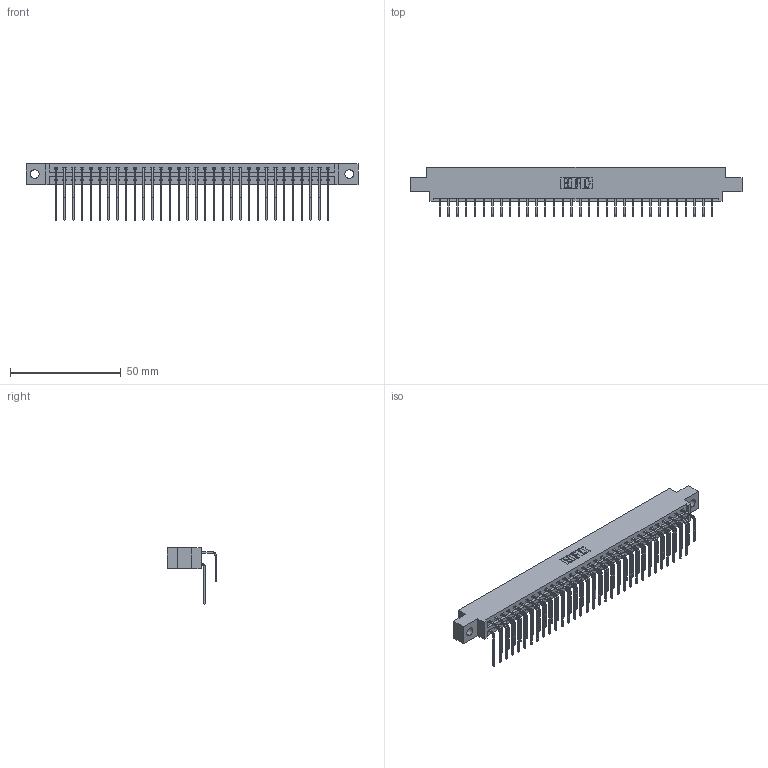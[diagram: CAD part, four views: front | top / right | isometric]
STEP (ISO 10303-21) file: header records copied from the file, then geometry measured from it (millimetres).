
FILE_DESCRIPTION (( 'STEP AP203' ), '1' );
FILE_NAME ('387-064-558-804.STEP', '2019-10-19T17:33:50', ( '' ), ( '' ), 'SwSTEP 2.0', 'SolidWorks 2016', '' );
FILE_SCHEMA (( 'CONFIG_CONTROL_DESIGN' ));
Length unit declared in the file: inch
Products named in the file (4): 345-292-001_558 559 Tail - 1; 387-064-558-804; 345-292-001_558 Tail - 2; 337 Part_0.170 Offset - 0.156 Dia-TH
Assembly tree (65 placements, depth 2):
  387-064-558-804
    337 Part_0.170 Offset - 0.156 Dia-TH
    345-292-001_558 559 Tail - 1  x32
    345-292-001_558 Tail - 2  x32
Bounding box: 149.81 x 22.17 x 25.53 mm (x, y, z)
Volume: 15818.8 mm3; surface area: 19545.1 mm2
Topology: 65 solids, 65 shells, 3702 faces, 11011 edges, 7254 vertices
Faces by surface type: plane 2634, cylinder 1068
Entity records: 28023 total; most frequent: CARTESIAN_POINT 4777, ORIENTED_EDGE 4662, DIRECTION 4063, EDGE_CURVE 2331, VECTOR 2163, LINE 2163, VERTEX_POINT 1550, AXIS2_PLACEMENT_3D 950
